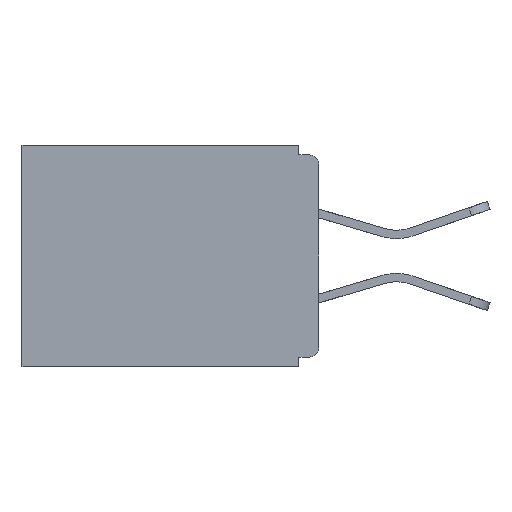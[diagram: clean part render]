
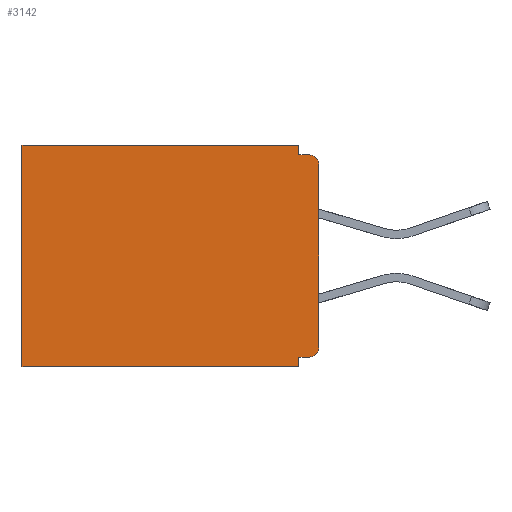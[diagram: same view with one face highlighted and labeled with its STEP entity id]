
A CAD part, left-side view. The second image highlights one B-rep face of the part: STEP entity #3142.
In plain terms, the highlighted planar face has unit normal (-1, 0, 0).
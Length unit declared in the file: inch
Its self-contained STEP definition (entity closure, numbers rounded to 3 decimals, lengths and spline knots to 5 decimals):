
#292 = CARTESIAN_POINT ( 'NONE',  ( 0.298, 0.031, -0.343 ) ) ;
#328 = EDGE_CURVE ( 'NONE', #8067, #2430, #1780, .T. ) ;
#329 = CARTESIAN_POINT ( 'NONE',  ( 0.298, 0., -0.328 ) ) ;
#782 = DIRECTION ( 'NONE',  ( 0., 0., -1. ) ) ;
#846 = DIRECTION ( 'NONE',  ( 0., -1., 0. ) ) ;
#1071 = CARTESIAN_POINT ( 'NONE',  ( 0.298, 0.015, -0.313 ) ) ;
#1208 = CARTESIAN_POINT ( 'NONE',  ( 0.298, 0., 0. ) ) ;
#1280 = CARTESIAN_POINT ( 'NONE',  ( 0.298, 0., 0. ) ) ;
#1290 = DIRECTION ( 'NONE',  ( 0., 0., -1. ) ) ;
#1304 = DIRECTION ( 'NONE',  ( 0., 1., 0. ) ) ;
#1341 = EDGE_CURVE ( 'NONE', #7307, #4329, #1485, .T. ) ;
#1485 = CIRCLE ( 'NONE', #7033, 0.015 ) ;
#1563 = CARTESIAN_POINT ( 'NONE',  ( 0.298, 0.031, 0. ) ) ;
#1592 = CARTESIAN_POINT ( 'NONE',  ( 0.298, 0.015, -0.03 ) ) ;
#1627 = EDGE_CURVE ( 'NONE', #5936, #10945, #3262, .T. ) ;
#1646 = DIRECTION ( 'NONE',  ( 0., 1., 0. ) ) ;
#1671 = CARTESIAN_POINT ( 'NONE',  ( 0.298, 0.46, 0. ) ) ;
#1766 = VERTEX_POINT ( 'NONE', #1671 ) ;
#1780 = LINE ( 'NONE', #4406, #7623 ) ;
#2098 = DIRECTION ( 'NONE',  ( 0., 0., -1. ) ) ;
#2166 = DIRECTION ( 'NONE',  ( 0., 0., -1. ) ) ;
#2221 = CARTESIAN_POINT ( 'NONE',  ( 0.298, 0.015, -0.328 ) ) ;
#2243 = CARTESIAN_POINT ( 'NONE',  ( 0.298, 0.46, -0.343 ) ) ;
#2321 = LINE ( 'NONE', #10396, #4766 ) ;
#2430 = VERTEX_POINT ( 'NONE', #2243 ) ;
#2488 = CARTESIAN_POINT ( 'NONE',  ( 0.298, 0.46, 0. ) ) ;
#2631 = DIRECTION ( 'NONE',  ( 0., 1., 0. ) ) ;
#2968 = LINE ( 'NONE', #3816, #5957 ) ;
#3142 = ADVANCED_FACE ( 'NONE', ( #9117 ), #6489, .F. ) ;
#3255 = ORIENTED_EDGE ( 'NONE', *, *, #5357, .F. ) ;
#3262 = LINE ( 'NONE', #329, #5032 ) ;
#3362 = LINE ( 'NONE', #5983, #6880 ) ;
#3515 = CARTESIAN_POINT ( 'NONE',  ( 0.298, 0., -0.03 ) ) ;
#3630 = VECTOR ( 'NONE', #2098, 39.37008 ) ;
#3816 = CARTESIAN_POINT ( 'NONE',  ( 0.298, 0.031, -0.343 ) ) ;
#4128 = EDGE_LOOP ( 'NONE', ( #6870, #3255, #5093, #4217, #10123, #8569, #7828, #7645, #6296, #9980 ) ) ;
#4217 = ORIENTED_EDGE ( 'NONE', *, *, #7219, .T. ) ;
#4329 = VERTEX_POINT ( 'NONE', #8202 ) ;
#4406 = CARTESIAN_POINT ( 'NONE',  ( 0.298, 0., -0.343 ) ) ;
#4766 = VECTOR ( 'NONE', #846, 39.37008 ) ;
#4808 = CIRCLE ( 'NONE', #8909, 0.015 ) ;
#5032 = VECTOR ( 'NONE', #1304, 39.37008 ) ;
#5093 = ORIENTED_EDGE ( 'NONE', *, *, #6350, .F. ) ;
#5144 = DIRECTION ( 'NONE',  ( 0., 0., -1. ) ) ;
#5357 = EDGE_CURVE ( 'NONE', #7242, #4329, #2321, .T. ) ;
#5539 = DIRECTION ( 'NONE',  ( 0., 0., -1. ) ) ;
#5706 = CARTESIAN_POINT ( 'NONE',  ( 0.298, 0.031, -0.343 ) ) ;
#5935 = LINE ( 'NONE', #5706, #9711 ) ;
#5936 = VERTEX_POINT ( 'NONE', #2221 ) ;
#5957 = VECTOR ( 'NONE', #9878, 39.37008 ) ;
#5983 = CARTESIAN_POINT ( 'NONE',  ( 0.298, 0., 0. ) ) ;
#6296 = ORIENTED_EDGE ( 'NONE', *, *, #11066, .T. ) ;
#6350 = EDGE_CURVE ( 'NONE', #7763, #7242, #2968, .T. ) ;
#6461 = AXIS2_PLACEMENT_3D ( 'NONE', #1280, #7344, #2166 ) ;
#6489 = PLANE ( 'NONE',  #6461 ) ;
#6609 = LINE ( 'NONE', #1208, #3630 ) ;
#6792 = DIRECTION ( 'NONE',  ( -1., 0., 0. ) ) ;
#6870 = ORIENTED_EDGE ( 'NONE', *, *, #1341, .T. ) ;
#6880 = VECTOR ( 'NONE', #1646, 39.37008 ) ;
#6940 = VERTEX_POINT ( 'NONE', #7300 ) ;
#7033 = AXIS2_PLACEMENT_3D ( 'NONE', #1592, #6792, #782 ) ;
#7219 = EDGE_CURVE ( 'NONE', #7763, #1766, #3362, .T. ) ;
#7242 = VERTEX_POINT ( 'NONE', #9453 ) ;
#7300 = CARTESIAN_POINT ( 'NONE',  ( 0.298, 0., -0.313 ) ) ;
#7307 = VERTEX_POINT ( 'NONE', #3515 ) ;
#7344 = DIRECTION ( 'NONE',  ( 1., 0., 0. ) ) ;
#7534 = EDGE_CURVE ( 'NONE', #10945, #8067, #5935, .T. ) ;
#7623 = VECTOR ( 'NONE', #2631, 39.37008 ) ;
#7645 = ORIENTED_EDGE ( 'NONE', *, *, #1627, .F. ) ;
#7763 = VERTEX_POINT ( 'NONE', #1563 ) ;
#7828 = ORIENTED_EDGE ( 'NONE', *, *, #7534, .F. ) ;
#8067 = VERTEX_POINT ( 'NONE', #292 ) ;
#8202 = CARTESIAN_POINT ( 'NONE',  ( 0.298, 0.015, -0.015 ) ) ;
#8569 = ORIENTED_EDGE ( 'NONE', *, *, #328, .F. ) ;
#8756 = LINE ( 'NONE', #2488, #10504 ) ;
#8841 = EDGE_CURVE ( 'NONE', #7307, #6940, #6609, .T. ) ;
#8885 = DIRECTION ( 'NONE',  ( -1., 0., 0. ) ) ;
#8909 = AXIS2_PLACEMENT_3D ( 'NONE', #1071, #8885, #5539 ) ;
#9104 = EDGE_CURVE ( 'NONE', #1766, #2430, #8756, .T. ) ;
#9117 = FACE_OUTER_BOUND ( 'NONE', #4128, .T. ) ;
#9453 = CARTESIAN_POINT ( 'NONE',  ( 0.298, 0.031, -0.015 ) ) ;
#9711 = VECTOR ( 'NONE', #1290, 39.37008 ) ;
#9878 = DIRECTION ( 'NONE',  ( 0., 0., -1. ) ) ;
#9980 = ORIENTED_EDGE ( 'NONE', *, *, #8841, .F. ) ;
#10123 = ORIENTED_EDGE ( 'NONE', *, *, #9104, .T. ) ;
#10396 = CARTESIAN_POINT ( 'NONE',  ( 0.298, 0., -0.015 ) ) ;
#10504 = VECTOR ( 'NONE', #5144, 39.37008 ) ;
#10945 = VERTEX_POINT ( 'NONE', #11064 ) ;
#11064 = CARTESIAN_POINT ( 'NONE',  ( 0.298, 0.031, -0.328 ) ) ;
#11066 = EDGE_CURVE ( 'NONE', #5936, #6940, #4808, .T. ) ;
